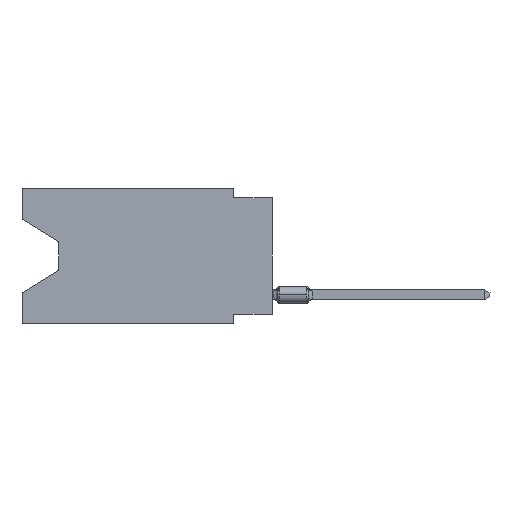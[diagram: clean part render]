
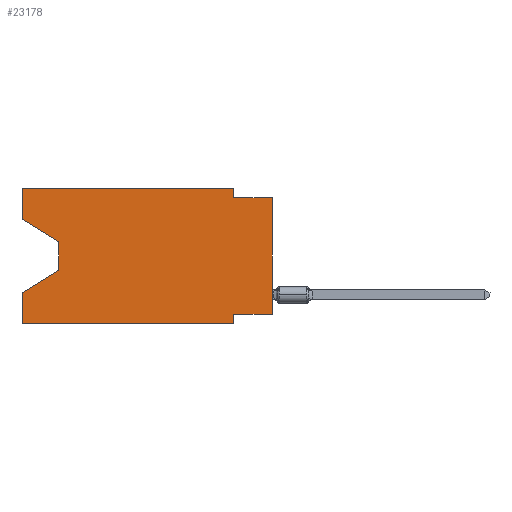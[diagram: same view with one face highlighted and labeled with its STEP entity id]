
A CAD part, left-side view. The second image highlights one B-rep face of the part: STEP entity #23178.
In plain terms, the highlighted planar face has unit normal (-1, 0, 0).
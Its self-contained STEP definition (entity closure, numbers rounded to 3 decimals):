
#204 = VECTOR ( 'NONE', #10386, 1000. ) ;
#390 = LINE ( 'NONE', #23599, #6015 ) ;
#585 = DIRECTION ( 'NONE',  ( 0., 0., -1. ) ) ;
#745 = PLANE ( 'NONE',  #16050 ) ;
#951 = CARTESIAN_POINT ( 'NONE',  ( 0., 0., -0.635 ) ) ;
#1191 = CARTESIAN_POINT ( 'NONE',  ( 0., 13.97, -3.505 ) ) ;
#1713 = VECTOR ( 'NONE', #19998, 1000. ) ;
#2253 = EDGE_CURVE ( 'NONE', #13449, #22070, #19330, .T. ) ;
#2438 = LINE ( 'NONE', #2729, #18585 ) ;
#2475 = CARTESIAN_POINT ( 'NONE',  ( 0., 2.54, -8.89 ) ) ;
#2476 = ORIENTED_EDGE ( 'NONE', *, *, #18016, .T. ) ;
#2729 = CARTESIAN_POINT ( 'NONE',  ( 0., 16.383, 0. ) ) ;
#2930 = VERTEX_POINT ( 'NONE', #28046 ) ;
#3323 = CARTESIAN_POINT ( 'NONE',  ( 0., 16.383, -8.89 ) ) ;
#3488 = CARTESIAN_POINT ( 'NONE',  ( 0., 16.383, 0. ) ) ;
#3499 = CARTESIAN_POINT ( 'NONE',  ( 0., 16.383, -2.038 ) ) ;
#3609 = ORIENTED_EDGE ( 'NONE', *, *, #9684, .F. ) ;
#4177 = CARTESIAN_POINT ( 'NONE',  ( 0., 13.97, -5.385 ) ) ;
#4343 = EDGE_CURVE ( 'NONE', #2930, #19155, #29098, .T. ) ;
#5067 = VECTOR ( 'NONE', #28847, 1000. ) ;
#5118 = EDGE_CURVE ( 'NONE', #27627, #22070, #29033, .T. ) ;
#5143 = CARTESIAN_POINT ( 'NONE',  ( 0., 2.54, -8.255 ) ) ;
#5211 = CARTESIAN_POINT ( 'NONE',  ( 0., 2.54, -0.635 ) ) ;
#5693 = VECTOR ( 'NONE', #24339, 1000. ) ;
#5779 = LINE ( 'NONE', #3499, #29924 ) ;
#6015 = VECTOR ( 'NONE', #21640, 1000. ) ;
#6058 = ORIENTED_EDGE ( 'NONE', *, *, #2253, .F. ) ;
#7621 = VECTOR ( 'NONE', #29247, 1000. ) ;
#8698 = EDGE_CURVE ( 'NONE', #10513, #2930, #5779, .T. ) ;
#8821 = ORIENTED_EDGE ( 'NONE', *, *, #8698, .T. ) ;
#9684 = EDGE_CURVE ( 'NONE', #17530, #22976, #29381, .T. ) ;
#9805 = DIRECTION ( 'NONE',  ( 0., 0., 1. ) ) ;
#10145 = EDGE_CURVE ( 'NONE', #19687, #13449, #12745, .T. ) ;
#10386 = DIRECTION ( 'NONE',  ( 0., 0., -1. ) ) ;
#10513 = VERTEX_POINT ( 'NONE', #19491 ) ;
#10776 = CARTESIAN_POINT ( 'NONE',  ( 0., 0., -8.255 ) ) ;
#11480 = VECTOR ( 'NONE', #24087, 1000. ) ;
#11935 = EDGE_CURVE ( 'NONE', #10513, #16137, #16952, .T. ) ;
#12125 = CARTESIAN_POINT ( 'NONE',  ( 0., 16.383, 0. ) ) ;
#12745 = LINE ( 'NONE', #10776, #23600 ) ;
#12781 = LINE ( 'NONE', #15508, #5067 ) ;
#12964 = LINE ( 'NONE', #26767, #204 ) ;
#13176 = EDGE_CURVE ( 'NONE', #19687, #22976, #14838, .T. ) ;
#13183 = ORIENTED_EDGE ( 'NONE', *, *, #13176, .T. ) ;
#13449 = VERTEX_POINT ( 'NONE', #5143 ) ;
#14838 = LINE ( 'NONE', #17113, #11480 ) ;
#14884 = ORIENTED_EDGE ( 'NONE', *, *, #11935, .F. ) ;
#15088 = CARTESIAN_POINT ( 'NONE',  ( 0., 2.54, -8.89 ) ) ;
#15172 = ORIENTED_EDGE ( 'NONE', *, *, #10145, .F. ) ;
#15192 = CARTESIAN_POINT ( 'NONE',  ( 0., 16.383, -6.852 ) ) ;
#15508 = CARTESIAN_POINT ( 'NONE',  ( 0., 13.97, -5.385 ) ) ;
#16050 = AXIS2_PLACEMENT_3D ( 'NONE', #12125, #26080, #585 ) ;
#16137 = VERTEX_POINT ( 'NONE', #3488 ) ;
#16532 = FACE_OUTER_BOUND ( 'NONE', #20313, .T. ) ;
#16952 = LINE ( 'NONE', #19212, #29024 ) ;
#17113 = CARTESIAN_POINT ( 'NONE',  ( 0., 0., 0. ) ) ;
#17357 = DIRECTION ( 'NONE',  ( 0., -1., 0. ) ) ;
#17530 = VERTEX_POINT ( 'NONE', #5211 ) ;
#17630 = EDGE_CURVE ( 'NONE', #21188, #17530, #12964, .T. ) ;
#18016 = EDGE_CURVE ( 'NONE', #19155, #26160, #12781, .T. ) ;
#18585 = VECTOR ( 'NONE', #27770, 1000. ) ;
#18915 = VECTOR ( 'NONE', #17357, 1000. ) ;
#18936 = ORIENTED_EDGE ( 'NONE', *, *, #28001, .F. ) ;
#19155 = VERTEX_POINT ( 'NONE', #4177 ) ;
#19212 = CARTESIAN_POINT ( 'NONE',  ( 0., 16.383, 0. ) ) ;
#19330 = LINE ( 'NONE', #15088, #5693 ) ;
#19491 = CARTESIAN_POINT ( 'NONE',  ( 0., 16.383, -2.038 ) ) ;
#19509 = CARTESIAN_POINT ( 'NONE',  ( 0., 0., -8.255 ) ) ;
#19687 = VERTEX_POINT ( 'NONE', #19509 ) ;
#19998 = DIRECTION ( 'NONE',  ( 0., -1., 0. ) ) ;
#20313 = EDGE_LOOP ( 'NONE', ( #8821, #25756, #2476, #21046, #21337, #6058, #15172, #13183, #3609, #22310, #18936, #14884 ) ) ;
#21046 = ORIENTED_EDGE ( 'NONE', *, *, #25993, .F. ) ;
#21188 = VERTEX_POINT ( 'NONE', #29100 ) ;
#21337 = ORIENTED_EDGE ( 'NONE', *, *, #5118, .T. ) ;
#21640 = DIRECTION ( 'NONE',  ( 0., -1., 0. ) ) ;
#21908 = CARTESIAN_POINT ( 'NONE',  ( 0., 16.383, -8.89 ) ) ;
#22070 = VERTEX_POINT ( 'NONE', #2475 ) ;
#22153 = DIRECTION ( 'NONE',  ( 0., 1., 0. ) ) ;
#22310 = ORIENTED_EDGE ( 'NONE', *, *, #17630, .F. ) ;
#22976 = VERTEX_POINT ( 'NONE', #951 ) ;
#23178 = ADVANCED_FACE ( 'NONE', ( #16532 ), #745, .F. ) ;
#23599 = CARTESIAN_POINT ( 'NONE',  ( 0., 16.383, 0. ) ) ;
#23600 = VECTOR ( 'NONE', #22153, 1000. ) ;
#24087 = DIRECTION ( 'NONE',  ( 0., 0., 1. ) ) ;
#24339 = DIRECTION ( 'NONE',  ( 0., 0., -1. ) ) ;
#25756 = ORIENTED_EDGE ( 'NONE', *, *, #4343, .T. ) ;
#25993 = EDGE_CURVE ( 'NONE', #27627, #26160, #2438, .T. ) ;
#26080 = DIRECTION ( 'NONE',  ( 1., 0., 0. ) ) ;
#26160 = VERTEX_POINT ( 'NONE', #15192 ) ;
#26767 = CARTESIAN_POINT ( 'NONE',  ( 0., 2.54, 0. ) ) ;
#26823 = CARTESIAN_POINT ( 'NONE',  ( 0., 0., -0.635 ) ) ;
#26873 = DIRECTION ( 'NONE',  ( 0., -0.855, -0.519 ) ) ;
#27627 = VERTEX_POINT ( 'NONE', #3323 ) ;
#27770 = DIRECTION ( 'NONE',  ( 0., 0., 1. ) ) ;
#28001 = EDGE_CURVE ( 'NONE', #16137, #21188, #390, .T. ) ;
#28046 = CARTESIAN_POINT ( 'NONE',  ( 0., 13.97, -3.505 ) ) ;
#28847 = DIRECTION ( 'NONE',  ( 0., 0.855, -0.519 ) ) ;
#29024 = VECTOR ( 'NONE', #9805, 1000. ) ;
#29033 = LINE ( 'NONE', #21908, #18915 ) ;
#29098 = LINE ( 'NONE', #1191, #7621 ) ;
#29100 = CARTESIAN_POINT ( 'NONE',  ( 0., 2.54, 0. ) ) ;
#29247 = DIRECTION ( 'NONE',  ( 0., 0., -1. ) ) ;
#29381 = LINE ( 'NONE', #26823, #1713 ) ;
#29924 = VECTOR ( 'NONE', #26873, 1000. ) ;
